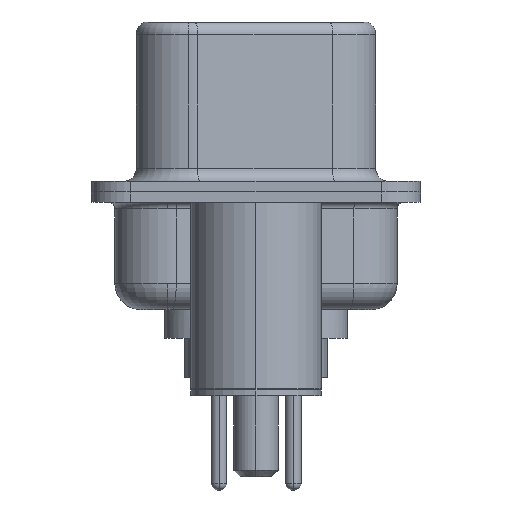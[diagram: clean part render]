
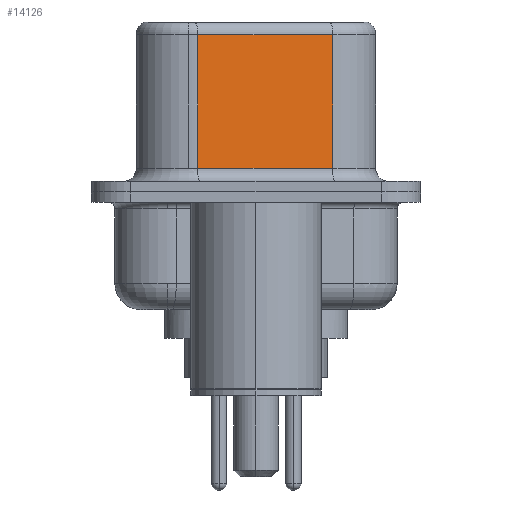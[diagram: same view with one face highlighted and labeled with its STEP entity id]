
A CAD part, left-side view. The second image highlights one B-rep face of the part: STEP entity #14126.
In plain terms, the highlighted planar face has unit normal (-0.985, -0.174, 0).
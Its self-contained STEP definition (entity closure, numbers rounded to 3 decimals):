
#121 = EDGE_CURVE ( 'NONE', #10145, #1322, #17607, .T. ) ;
#361 = CARTESIAN_POINT ( 'NONE',  ( 4.585, -2.927, 6.52 ) ) ;
#570 = ORIENTED_EDGE ( 'NONE', *, *, #16089, .T. ) ;
#1322 = VERTEX_POINT ( 'NONE', #9427 ) ;
#1564 = PLANE ( 'NONE',  #2795 ) ;
#1779 = CARTESIAN_POINT ( 'NONE',  ( 4.585, -2.927, 6.02 ) ) ;
#2191 = LINE ( 'NONE', #1779, #16345 ) ;
#2795 = AXIS2_PLACEMENT_3D ( 'NONE', #10996, #7009, #16670 ) ;
#2989 = VECTOR ( 'NONE', #6873, 1000. ) ;
#3136 = DIRECTION ( 'NONE',  ( -0.174, 0.985, 0. ) ) ;
#3323 = ORIENTED_EDGE ( 'NONE', *, *, #11596, .T. ) ;
#6329 = EDGE_LOOP ( 'NONE', ( #13262, #16461, #3323, #570 ) ) ;
#6585 = EDGE_CURVE ( 'NONE', #10145, #8487, #2191, .T. ) ;
#6700 = CARTESIAN_POINT ( 'NONE',  ( 3.675, 2.233, 0.9 ) ) ;
#6873 = DIRECTION ( 'NONE',  ( 0.174, -0.985, 0. ) ) ;
#7009 = DIRECTION ( 'NONE',  ( 0.985, 0.174, 0. ) ) ;
#7014 = VECTOR ( 'NONE', #7382, 1000. ) ;
#7184 = CARTESIAN_POINT ( 'NONE',  ( 3.675, 2.233, 6.52 ) ) ;
#7382 = DIRECTION ( 'NONE',  ( 0., 0., -1. ) ) ;
#8487 = VERTEX_POINT ( 'NONE', #16766 ) ;
#9427 = CARTESIAN_POINT ( 'NONE',  ( 4.585, -2.927, 0.9 ) ) ;
#9941 = FACE_OUTER_BOUND ( 'NONE', #6329, .T. ) ;
#10145 = VERTEX_POINT ( 'NONE', #16172 ) ;
#10878 = LINE ( 'NONE', #7184, #15044 ) ;
#10996 = CARTESIAN_POINT ( 'NONE',  ( 4.585, -2.927, 6.52 ) ) ;
#11596 = EDGE_CURVE ( 'NONE', #8487, #11812, #10878, .T. ) ;
#11812 = VERTEX_POINT ( 'NONE', #6700 ) ;
#13262 = ORIENTED_EDGE ( 'NONE', *, *, #121, .F. ) ;
#13785 = LINE ( 'NONE', #16544, #2989 ) ;
#14126 = ADVANCED_FACE ( 'NONE', ( #9941 ), #1564, .F. ) ;
#15044 = VECTOR ( 'NONE', #16851, 1000. ) ;
#16089 = EDGE_CURVE ( 'NONE', #11812, #1322, #13785, .T. ) ;
#16172 = CARTESIAN_POINT ( 'NONE',  ( 4.585, -2.927, 6.02 ) ) ;
#16345 = VECTOR ( 'NONE', #3136, 1000. ) ;
#16461 = ORIENTED_EDGE ( 'NONE', *, *, #6585, .T. ) ;
#16544 = CARTESIAN_POINT ( 'NONE',  ( 4.585, -2.927, 0.9 ) ) ;
#16670 = DIRECTION ( 'NONE',  ( -0.174, 0.985, 0. ) ) ;
#16766 = CARTESIAN_POINT ( 'NONE',  ( 3.675, 2.233, 6.02 ) ) ;
#16851 = DIRECTION ( 'NONE',  ( 0., 0., -1. ) ) ;
#17607 = LINE ( 'NONE', #361, #7014 ) ;
